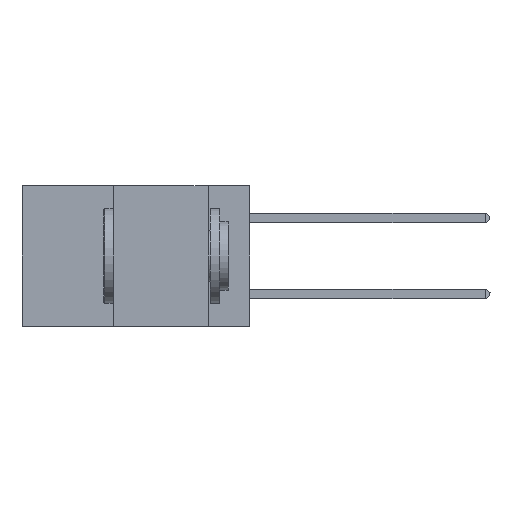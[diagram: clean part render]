
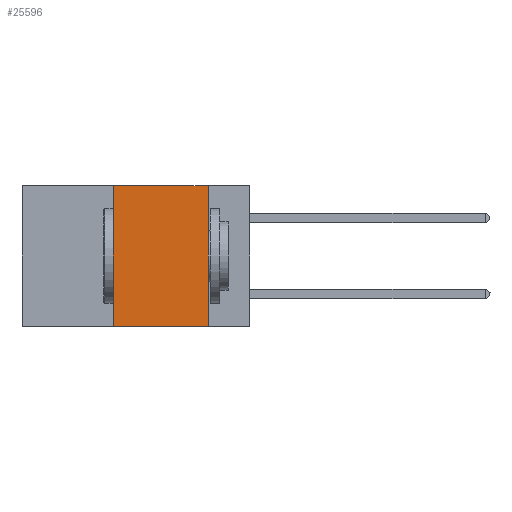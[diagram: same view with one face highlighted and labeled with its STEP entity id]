
A CAD part, left-side view. The second image highlights one B-rep face of the part: STEP entity #25596.
In plain terms, the highlighted planar face has unit normal (-1, 0, 0).
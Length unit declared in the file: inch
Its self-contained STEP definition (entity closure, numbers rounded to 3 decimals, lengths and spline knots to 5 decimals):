
#1036 = ORIENTED_EDGE ( 'NONE', *, *, #16272, .T. ) ;
#1692 = LINE ( 'NONE', #6342, #24607 ) ;
#2230 = DIRECTION ( 'NONE',  ( 0., 0., -1. ) ) ;
#2879 = CARTESIAN_POINT ( 'NONE',  ( 0., 0.11, -0.37 ) ) ;
#4411 = CARTESIAN_POINT ( 'NONE',  ( 0., 0.36, 0. ) ) ;
#5301 = EDGE_LOOP ( 'NONE', ( #22105, #11457, #7186, #1036 ) ) ;
#5827 = EDGE_CURVE ( 'NONE', #12626, #19538, #1692, .T. ) ;
#6342 = CARTESIAN_POINT ( 'NONE',  ( 0., 0.11, 0. ) ) ;
#7186 = ORIENTED_EDGE ( 'NONE', *, *, #15929, .F. ) ;
#9231 = CARTESIAN_POINT ( 'NONE',  ( 0., 0.36, 0. ) ) ;
#10652 = LINE ( 'NONE', #17702, #13808 ) ;
#11457 = ORIENTED_EDGE ( 'NONE', *, *, #19420, .F. ) ;
#11985 = VERTEX_POINT ( 'NONE', #24153 ) ;
#12626 = VERTEX_POINT ( 'NONE', #14301 ) ;
#13808 = VECTOR ( 'NONE', #15427, 39.37008 ) ;
#14282 = VERTEX_POINT ( 'NONE', #4411 ) ;
#14301 = CARTESIAN_POINT ( 'NONE',  ( 0., 0.11, 0. ) ) ;
#15427 = DIRECTION ( 'NONE',  ( 0., -1., 0. ) ) ;
#15440 = CARTESIAN_POINT ( 'NONE',  ( 0., 0.6, 0. ) ) ;
#15929 = EDGE_CURVE ( 'NONE', #11985, #14282, #17256, .T. ) ;
#16272 = EDGE_CURVE ( 'NONE', #11985, #19538, #10652, .T. ) ;
#17256 = LINE ( 'NONE', #9231, #25430 ) ;
#17285 = DIRECTION ( 'NONE',  ( 0., 0., 1. ) ) ;
#17702 = CARTESIAN_POINT ( 'NONE',  ( 0., 0.6, -0.37 ) ) ;
#17891 = CARTESIAN_POINT ( 'NONE',  ( 0., 0.6, 0. ) ) ;
#18164 = DIRECTION ( 'NONE',  ( 1., 0., 0. ) ) ;
#18438 = AXIS2_PLACEMENT_3D ( 'NONE', #17891, #18164, #24212 ) ;
#18809 = VECTOR ( 'NONE', #23129, 39.37008 ) ;
#19420 = EDGE_CURVE ( 'NONE', #14282, #12626, #24117, .T. ) ;
#19538 = VERTEX_POINT ( 'NONE', #2879 ) ;
#20413 = FACE_OUTER_BOUND ( 'NONE', #5301, .T. ) ;
#22105 = ORIENTED_EDGE ( 'NONE', *, *, #5827, .F. ) ;
#22190 = PLANE ( 'NONE',  #18438 ) ;
#23129 = DIRECTION ( 'NONE',  ( 0., -1., 0. ) ) ;
#24117 = LINE ( 'NONE', #15440, #18809 ) ;
#24153 = CARTESIAN_POINT ( 'NONE',  ( 0., 0.36, -0.37 ) ) ;
#24212 = DIRECTION ( 'NONE',  ( 0., 0., -1. ) ) ;
#24607 = VECTOR ( 'NONE', #2230, 39.37008 ) ;
#25430 = VECTOR ( 'NONE', #17285, 39.37008 ) ;
#25596 = ADVANCED_FACE ( 'NONE', ( #20413 ), #22190, .F. ) ;
